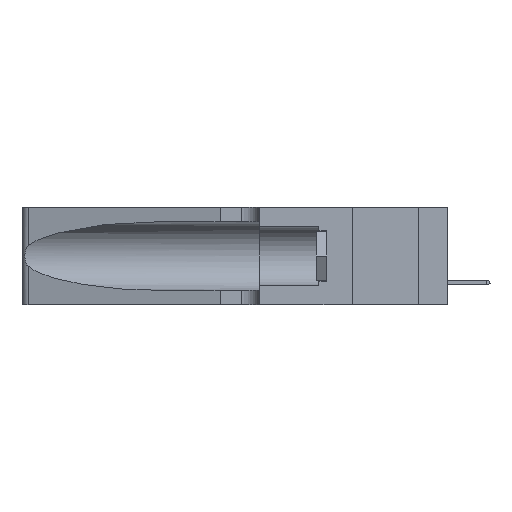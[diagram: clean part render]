
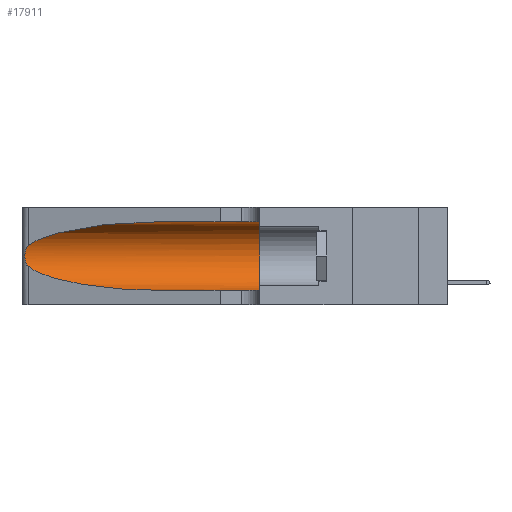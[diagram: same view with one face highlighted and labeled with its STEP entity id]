
A CAD part, left-side view. The second image highlights one B-rep face of the part: STEP entity #17911.
In plain terms, the highlighted cylindrical face has radius 3.308 mm (diameter 6.617 mm), a partial arc.
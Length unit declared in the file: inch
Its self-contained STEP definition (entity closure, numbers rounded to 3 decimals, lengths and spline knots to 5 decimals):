
#164 = EDGE_CURVE ( 'NONE', #5134, #20889, #391, .T. ) ;
#391 =( BOUNDED_CURVE ( )  B_SPLINE_CURVE ( 3, ( #27659, #3597, #23105, #16512 ),
 .UNSPECIFIED., .F., .T. ) 
 B_SPLINE_CURVE_WITH_KNOTS ( ( 4, 4 ),
 ( 1.5708, 2.84003 ),
 .UNSPECIFIED. ) 
 CURVE ( )  GEOMETRIC_REPRESENTATION_ITEM ( )  RATIONAL_B_SPLINE_CURVE ( ( 1., 0.87, 0.87, 1. ) ) 
 REPRESENTATION_ITEM ( '' )  );
#448 = CARTESIAN_POINT ( 'NONE',  ( 0.25789, 1.23486, 0.15765 ) ) ;
#637 = CARTESIAN_POINT ( 'NONE',  ( 0.26018, 1.23835, 0.19895 ) ) ;
#1885 = ORIENTED_EDGE ( 'NONE', *, *, #11567, .T. ) ;
#1966 = VECTOR ( 'NONE', #12558, 39.37008 ) ;
#2496 = EDGE_CURVE ( 'NONE', #19829, #12271, #6350, .T. ) ;
#2555 = EDGE_LOOP ( 'NONE', ( #12328, #1885, #21987, #18891, #13665, #25502 ) ) ;
#2684 = CARTESIAN_POINT ( 'NONE',  ( 0.1305, 1.61858, 0.185 ) ) ;
#2769 = CARTESIAN_POINT ( 'NONE',  ( 0.25487, 1.22718, 0.22369 ) ) ;
#3293 = CARTESIAN_POINT ( 'NONE',  ( 0.1305, 1.61858, 0.31525 ) ) ;
#3581 = VERTEX_POINT ( 'NONE', #11072 ) ;
#3597 = CARTESIAN_POINT ( 'NONE',  ( 0.18966, 0.96281, 0.31525 ) ) ;
#3716 = CARTESIAN_POINT ( 'NONE',  ( 0.25487, 1.22718, 0.22369 ) ) ;
#4276 = EDGE_CURVE ( 'NONE', #3581, #4316, #8843, .T. ) ;
#4316 = VERTEX_POINT ( 'NONE', #8231 ) ;
#4896 = CARTESIAN_POINT ( 'NONE',  ( 0.25555, 1.22993, 0.14849 ) ) ;
#5134 = VERTEX_POINT ( 'NONE', #11751 ) ;
#5179 = CARTESIAN_POINT ( 'NONE',  ( 0.25856, 1.23593, 0.16098 ) ) ;
#6350 = CIRCLE ( 'NONE', #22642, 0.13025 ) ;
#7188 = CARTESIAN_POINT ( 'NONE',  ( 0.25487, 1.22718, 0.14631 ) ) ;
#8231 = CARTESIAN_POINT ( 'NONE',  ( 0.1305, 0.72297, 0.05475 ) ) ;
#8843 =( BOUNDED_CURVE ( )  B_SPLINE_CURVE ( 3, ( #9801, #25109, #11977, #16406 ),
 .UNSPECIFIED., .F., .T. ) 
 B_SPLINE_CURVE_WITH_KNOTS ( ( 4, 4 ),
 ( 3.44316, 4.71239 ),
 .UNSPECIFIED. ) 
 CURVE ( )  GEOMETRIC_REPRESENTATION_ITEM ( )  RATIONAL_B_SPLINE_CURVE ( ( 1., 0.87, 0.87, 1. ) ) 
 REPRESENTATION_ITEM ( '' )  );
#9194 = CARTESIAN_POINT ( 'NONE',  ( 0.25555, 1.22994, 0.2215 ) ) ;
#9371 = CARTESIAN_POINT ( 'NONE',  ( 0.25787, 1.23484, 0.2124 ) ) ;
#9801 = CARTESIAN_POINT ( 'NONE',  ( 0.25487, 1.22718, 0.14631 ) ) ;
#10421 = DIRECTION ( 'NONE',  ( 0., 1., 0. ) ) ;
#11064 = VECTOR ( 'NONE', #16491, 39.37008 ) ;
#11072 = CARTESIAN_POINT ( 'NONE',  ( 0.25487, 1.22718, 0.14631 ) ) ;
#11567 = EDGE_CURVE ( 'NONE', #20889, #3581, #16906, .T. ) ;
#11632 = CARTESIAN_POINT ( 'NONE',  ( 0.25639, 1.23186, 0.15144 ) ) ;
#11751 = CARTESIAN_POINT ( 'NONE',  ( 0.1305, 0.72297, 0.31525 ) ) ;
#11977 = CARTESIAN_POINT ( 'NONE',  ( 0.18966, 0.96281, 0.05475 ) ) ;
#12271 = VERTEX_POINT ( 'NONE', #14851 ) ;
#12328 = ORIENTED_EDGE ( 'NONE', *, *, #164, .T. ) ;
#12476 = LINE ( 'NONE', #3293, #11064 ) ;
#12558 = DIRECTION ( 'NONE',  ( 0., -1., 0. ) ) ;
#13593 = CARTESIAN_POINT ( 'NONE',  ( 0.25854, 1.2359, 0.20912 ) ) ;
#13665 = ORIENTED_EDGE ( 'NONE', *, *, #2496, .F. ) ;
#13882 = CARTESIAN_POINT ( 'NONE',  ( 0.26075, 1.23896, 0.19203 ) ) ;
#14708 = EDGE_CURVE ( 'NONE', #4316, #12271, #28373, .T. ) ;
#14851 = CARTESIAN_POINT ( 'NONE',  ( 0.1305, 0.35, 0.05475 ) ) ;
#15018 = DIRECTION ( 'NONE',  ( 0., 0., 1. ) ) ;
#16167 = DIRECTION ( 'NONE',  ( 0., 0., -1. ) ) ;
#16406 = CARTESIAN_POINT ( 'NONE',  ( 0.1305, 0.72297, 0.05475 ) ) ;
#16491 = DIRECTION ( 'NONE',  ( 0., -1., 0. ) ) ;
#16512 = CARTESIAN_POINT ( 'NONE',  ( 0.25487, 1.22718, 0.22369 ) ) ;
#16906 = B_SPLINE_CURVE_WITH_KNOTS ( 'NONE', 3,
 ( #2769, #9194, #24780, #9371, #13593, #637, #13882, #18342, #20525, #5179, #448, #11632, #4896, #7188 ),
 .UNSPECIFIED., .F., .F.,
 ( 4, 2, 2, 2, 2, 2, 4 ),
 ( 0., 0.00027, 0.00053, 0.00107, 0.0016, 0.00187, 0.00214 ),
 .UNSPECIFIED. ) ;
#17911 = ADVANCED_FACE ( 'NONE', ( #19443 ), #21841, .F. ) ;
#18342 = CARTESIAN_POINT ( 'NONE',  ( 0.26075, 1.23896, 0.178 ) ) ;
#18436 = DIRECTION ( 'NONE',  ( 0., -1., 0. ) ) ;
#18891 = ORIENTED_EDGE ( 'NONE', *, *, #14708, .T. ) ;
#19443 = FACE_OUTER_BOUND ( 'NONE', #2555, .T. ) ;
#19829 = VERTEX_POINT ( 'NONE', #26348 ) ;
#20092 = EDGE_CURVE ( 'NONE', #5134, #19829, #12476, .T. ) ;
#20525 = CARTESIAN_POINT ( 'NONE',  ( 0.26017, 1.23833, 0.17102 ) ) ;
#20889 = VERTEX_POINT ( 'NONE', #3716 ) ;
#21841 = CYLINDRICAL_SURFACE ( 'NONE', #22750, 0.13025 ) ;
#21987 = ORIENTED_EDGE ( 'NONE', *, *, #4276, .T. ) ;
#22642 = AXIS2_PLACEMENT_3D ( 'NONE', #23717, #10421, #15018 ) ;
#22750 = AXIS2_PLACEMENT_3D ( 'NONE', #2684, #18436, #16167 ) ;
#23105 = CARTESIAN_POINT ( 'NONE',  ( 0.2373, 1.15595, 0.28018 ) ) ;
#23717 = CARTESIAN_POINT ( 'NONE',  ( 0.1305, 0.35, 0.185 ) ) ;
#24780 = CARTESIAN_POINT ( 'NONE',  ( 0.25639, 1.23184, 0.21858 ) ) ;
#25109 = CARTESIAN_POINT ( 'NONE',  ( 0.2373, 1.15595, 0.08982 ) ) ;
#25502 = ORIENTED_EDGE ( 'NONE', *, *, #20092, .F. ) ;
#26348 = CARTESIAN_POINT ( 'NONE',  ( 0.1305, 0.35, 0.31525 ) ) ;
#27659 = CARTESIAN_POINT ( 'NONE',  ( 0.1305, 0.72297, 0.31525 ) ) ;
#28048 = CARTESIAN_POINT ( 'NONE',  ( 0.1305, 1.61858, 0.05475 ) ) ;
#28373 = LINE ( 'NONE', #28048, #1966 ) ;
